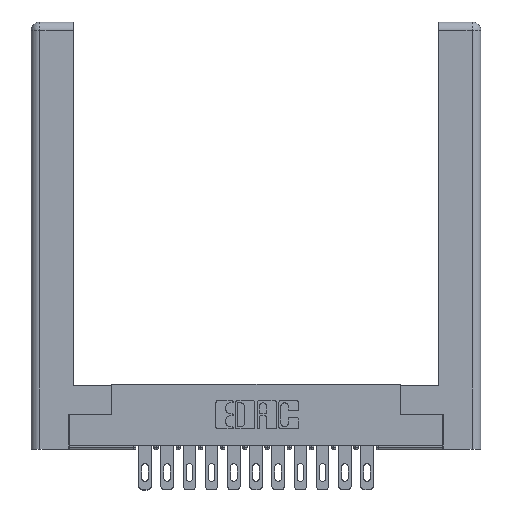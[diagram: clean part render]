
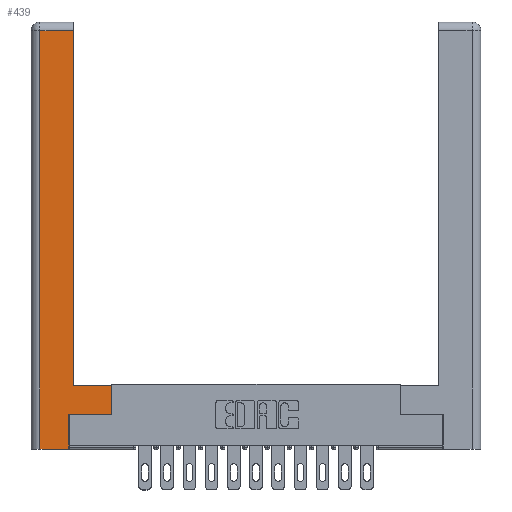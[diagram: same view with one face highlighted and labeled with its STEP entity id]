
A CAD part, top view. The second image highlights one B-rep face of the part: STEP entity #439.
In plain terms, the highlighted planar face has unit normal (0, 0, 1).
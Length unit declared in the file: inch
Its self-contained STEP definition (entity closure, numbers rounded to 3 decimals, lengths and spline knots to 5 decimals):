
#16 = CARTESIAN_POINT ( 'NONE',  ( 0.295, 0.45, 0. ) ) ;
#354 = DIRECTION ( 'NONE',  ( 0., 1., 0. ) ) ;
#439 = ADVANCED_FACE ( 'NONE', ( #16430 ), #9369, .F. ) ;
#887 = CARTESIAN_POINT ( 'NONE',  ( 0., 0., 0. ) ) ;
#935 = VECTOR ( 'NONE', #6862, 39.37008 ) ;
#1607 = VERTEX_POINT ( 'NONE', #12901 ) ;
#1686 = LINE ( 'NONE', #6979, #3928 ) ;
#2212 = ORIENTED_EDGE ( 'NONE', *, *, #4470, .T. ) ;
#2315 = DIRECTION ( 'NONE',  ( 0., 0., -1. ) ) ;
#2714 = DIRECTION ( 'NONE',  ( 0., -1., 0. ) ) ;
#2739 = DIRECTION ( 'NONE',  ( -1., 0., 0. ) ) ;
#3900 = EDGE_LOOP ( 'NONE', ( #2212, #13054, #9257, #8085, #17599, #14394, #13027, #5140 ) ) ;
#3928 = VECTOR ( 'NONE', #4230, 39.37008 ) ;
#4227 = VECTOR ( 'NONE', #2714, 39.37008 ) ;
#4230 = DIRECTION ( 'NONE',  ( 0., 1., 0. ) ) ;
#4470 = EDGE_CURVE ( 'NONE', #1607, #5625, #17651, .T. ) ;
#4925 = CARTESIAN_POINT ( 'NONE',  ( 0.265, 0., 0. ) ) ;
#4946 = LINE ( 'NONE', #8283, #935 ) ;
#5140 = ORIENTED_EDGE ( 'NONE', *, *, #14745, .T. ) ;
#5255 = VECTOR ( 'NONE', #354, 39.37008 ) ;
#5470 = DIRECTION ( 'NONE',  ( 1., 0., 0. ) ) ;
#5625 = VERTEX_POINT ( 'NONE', #13010 ) ;
#5878 = DIRECTION ( 'NONE',  ( 0., 1., 0. ) ) ;
#5982 = EDGE_CURVE ( 'NONE', #7843, #17836, #11285, .T. ) ;
#6862 = DIRECTION ( 'NONE',  ( -1., 0., 0. ) ) ;
#6979 = CARTESIAN_POINT ( 'NONE',  ( 0.265, 0.245, 0. ) ) ;
#7631 = LINE ( 'NONE', #11106, #18068 ) ;
#7802 = VECTOR ( 'NONE', #14791, 39.37008 ) ;
#7843 = VERTEX_POINT ( 'NONE', #17618 ) ;
#8085 = ORIENTED_EDGE ( 'NONE', *, *, #14876, .T. ) ;
#8283 = CARTESIAN_POINT ( 'NONE',  ( 0.0615, 2.94, 0. ) ) ;
#8660 = EDGE_CURVE ( 'NONE', #15092, #17221, #7631, .T. ) ;
#8699 = LINE ( 'NONE', #4925, #7802 ) ;
#9246 = AXIS2_PLACEMENT_3D ( 'NONE', #887, #2315, #2739 ) ;
#9257 = ORIENTED_EDGE ( 'NONE', *, *, #5982, .T. ) ;
#9369 = PLANE ( 'NONE',  #9246 ) ;
#9772 = CARTESIAN_POINT ( 'NONE',  ( 0.0615, 0., 0. ) ) ;
#10326 = EDGE_CURVE ( 'NONE', #5625, #7843, #4946, .T. ) ;
#11106 = CARTESIAN_POINT ( 'NONE',  ( 0.565, 0.245, 0. ) ) ;
#11285 = LINE ( 'NONE', #9772, #4227 ) ;
#11346 = CARTESIAN_POINT ( 'NONE',  ( 0.0615, 0., 0. ) ) ;
#12055 = LINE ( 'NONE', #16, #16454 ) ;
#12348 = CARTESIAN_POINT ( 'NONE',  ( 0.265, 0., 0. ) ) ;
#12447 = CARTESIAN_POINT ( 'NONE',  ( 0.265, 0.245, 0. ) ) ;
#12745 = VERTEX_POINT ( 'NONE', #16125 ) ;
#12807 = EDGE_CURVE ( 'NONE', #17221, #12745, #13461, .T. ) ;
#12901 = CARTESIAN_POINT ( 'NONE',  ( 0.295, 0.45, 0. ) ) ;
#13010 = CARTESIAN_POINT ( 'NONE',  ( 0.295, 2.94, 0. ) ) ;
#13027 = ORIENTED_EDGE ( 'NONE', *, *, #12807, .T. ) ;
#13054 = ORIENTED_EDGE ( 'NONE', *, *, #10326, .T. ) ;
#13108 = CARTESIAN_POINT ( 'NONE',  ( 0.565, 0.45, 0. ) ) ;
#13282 = EDGE_CURVE ( 'NONE', #13577, #15092, #1686, .T. ) ;
#13461 = LINE ( 'NONE', #13108, #5255 ) ;
#13577 = VERTEX_POINT ( 'NONE', #12348 ) ;
#14385 = DIRECTION ( 'NONE',  ( -1., 0., 0. ) ) ;
#14394 = ORIENTED_EDGE ( 'NONE', *, *, #8660, .T. ) ;
#14745 = EDGE_CURVE ( 'NONE', #12745, #1607, #12055, .T. ) ;
#14791 = DIRECTION ( 'NONE',  ( 1., 0., 0. ) ) ;
#14876 = EDGE_CURVE ( 'NONE', #17836, #13577, #8699, .T. ) ;
#15092 = VERTEX_POINT ( 'NONE', #12447 ) ;
#15709 = CARTESIAN_POINT ( 'NONE',  ( 0.295, 3., 0. ) ) ;
#16125 = CARTESIAN_POINT ( 'NONE',  ( 0.565, 0.45, 0. ) ) ;
#16295 = VECTOR ( 'NONE', #5878, 39.37008 ) ;
#16430 = FACE_OUTER_BOUND ( 'NONE', #3900, .T. ) ;
#16454 = VECTOR ( 'NONE', #14385, 39.37008 ) ;
#17221 = VERTEX_POINT ( 'NONE', #17271 ) ;
#17271 = CARTESIAN_POINT ( 'NONE',  ( 0.565, 0.245, 0. ) ) ;
#17599 = ORIENTED_EDGE ( 'NONE', *, *, #13282, .T. ) ;
#17618 = CARTESIAN_POINT ( 'NONE',  ( 0.0615, 2.94, 0. ) ) ;
#17651 = LINE ( 'NONE', #15709, #16295 ) ;
#17836 = VERTEX_POINT ( 'NONE', #11346 ) ;
#18068 = VECTOR ( 'NONE', #5470, 39.37008 ) ;
